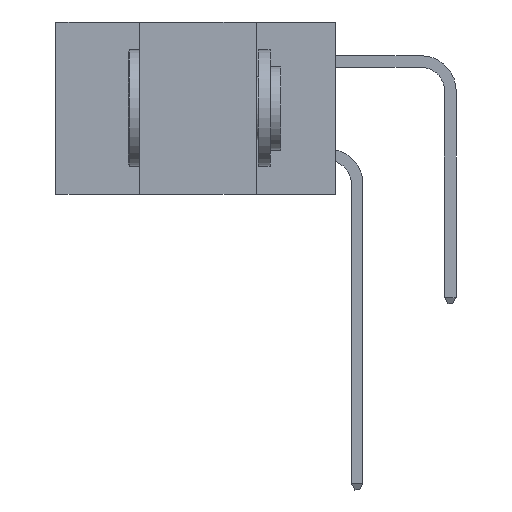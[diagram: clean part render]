
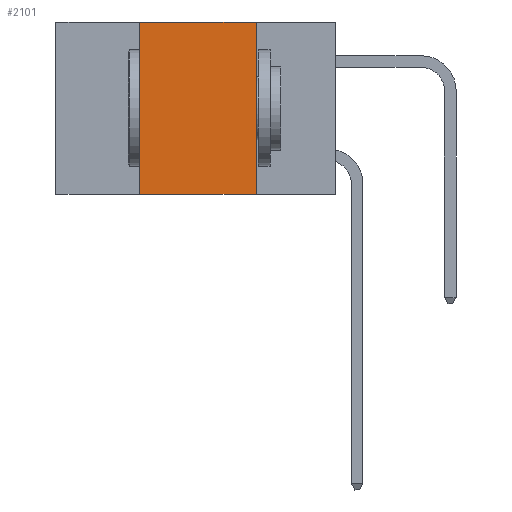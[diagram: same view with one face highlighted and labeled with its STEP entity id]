
A CAD part, left-side view. The second image highlights one B-rep face of the part: STEP entity #2101.
In plain terms, the highlighted planar face has unit normal (-1, 0, 0).
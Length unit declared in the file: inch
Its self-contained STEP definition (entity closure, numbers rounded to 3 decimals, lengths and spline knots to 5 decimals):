
#401 = EDGE_CURVE ( 'NONE', #5181, #12246, #5433, .T. ) ;
#636 = VERTEX_POINT ( 'NONE', #11697 ) ;
#1212 = VERTEX_POINT ( 'NONE', #5735 ) ;
#1632 = EDGE_CURVE ( 'NONE', #5181, #636, #9020, .T. ) ;
#2101 = ADVANCED_FACE ( 'NONE', ( #8650 ), #8302, .F. ) ;
#3089 = EDGE_LOOP ( 'NONE', ( #9847, #13560, #10851, #12524 ) ) ;
#3363 = EDGE_CURVE ( 'NONE', #12246, #1212, #13492, .T. ) ;
#3598 = DIRECTION ( 'NONE',  ( 0., 0., 1. ) ) ;
#5120 = CARTESIAN_POINT ( 'NONE',  ( 0., 0.17, 0. ) ) ;
#5181 = VERTEX_POINT ( 'NONE', #12625 ) ;
#5190 = CARTESIAN_POINT ( 'NONE',  ( 0., 0.42, 0. ) ) ;
#5227 = VECTOR ( 'NONE', #6187, 39.37008 ) ;
#5433 = LINE ( 'NONE', #7126, #13622 ) ;
#5735 = CARTESIAN_POINT ( 'NONE',  ( 0., 0.17, 0. ) ) ;
#5837 = VECTOR ( 'NONE', #6100, 39.37008 ) ;
#6100 = DIRECTION ( 'NONE',  ( 0., -1., 0. ) ) ;
#6187 = DIRECTION ( 'NONE',  ( 0., 0., -1. ) ) ;
#7126 = CARTESIAN_POINT ( 'NONE',  ( 0., 0.42, 0. ) ) ;
#7450 = AXIS2_PLACEMENT_3D ( 'NONE', #8334, #8739, #8163 ) ;
#7704 = CARTESIAN_POINT ( 'NONE',  ( 0., 0.6, 0. ) ) ;
#8059 = LINE ( 'NONE', #5120, #5227 ) ;
#8163 = DIRECTION ( 'NONE',  ( 0., 0., -1. ) ) ;
#8194 = CARTESIAN_POINT ( 'NONE',  ( 0., 0.6, -0.37 ) ) ;
#8302 = PLANE ( 'NONE',  #7450 ) ;
#8334 = CARTESIAN_POINT ( 'NONE',  ( 0., 0.6, 0. ) ) ;
#8650 = FACE_OUTER_BOUND ( 'NONE', #3089, .T. ) ;
#8739 = DIRECTION ( 'NONE',  ( 1., 0., 0. ) ) ;
#9020 = LINE ( 'NONE', #8194, #5837 ) ;
#9847 = ORIENTED_EDGE ( 'NONE', *, *, #11553, .F. ) ;
#10204 = DIRECTION ( 'NONE',  ( 0., -1., 0. ) ) ;
#10327 = VECTOR ( 'NONE', #10204, 39.37008 ) ;
#10851 = ORIENTED_EDGE ( 'NONE', *, *, #401, .F. ) ;
#11553 = EDGE_CURVE ( 'NONE', #1212, #636, #8059, .T. ) ;
#11697 = CARTESIAN_POINT ( 'NONE',  ( 0., 0.17, -0.37 ) ) ;
#12246 = VERTEX_POINT ( 'NONE', #5190 ) ;
#12524 = ORIENTED_EDGE ( 'NONE', *, *, #1632, .T. ) ;
#12625 = CARTESIAN_POINT ( 'NONE',  ( 0., 0.42, -0.37 ) ) ;
#13492 = LINE ( 'NONE', #7704, #10327 ) ;
#13560 = ORIENTED_EDGE ( 'NONE', *, *, #3363, .F. ) ;
#13622 = VECTOR ( 'NONE', #3598, 39.37008 ) ;
